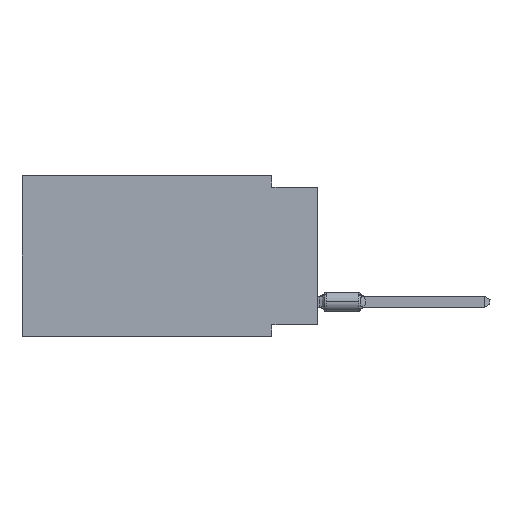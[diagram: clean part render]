
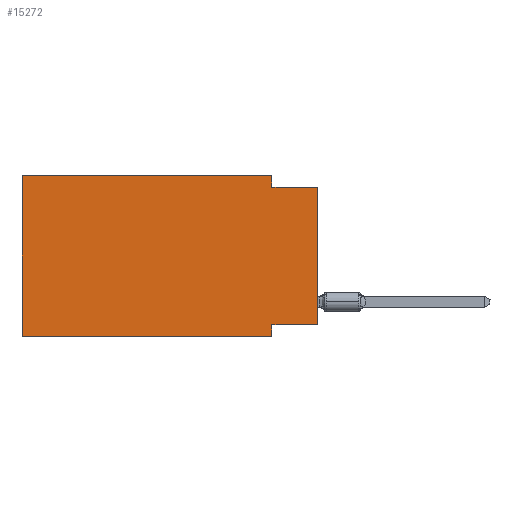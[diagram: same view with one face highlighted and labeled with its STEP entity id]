
A CAD part, left-side view. The second image highlights one B-rep face of the part: STEP entity #15272.
In plain terms, the highlighted planar face has unit normal (-1, 0, 0).
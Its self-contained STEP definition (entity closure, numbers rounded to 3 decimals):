
#421 = VECTOR ( 'NONE', #10780, 1000. ) ;
#685 = EDGE_CURVE ( 'NONE', #40255, #81278, #8906, .T. ) ;
#837 = ORIENTED_EDGE ( 'NONE', *, *, #5500, .F. ) ;
#1080 = VECTOR ( 'NONE', #57625, 1000. ) ;
#1341 = CARTESIAN_POINT ( 'NONE',  ( 0., 16.383, 0. ) ) ;
#1857 = ORIENTED_EDGE ( 'NONE', *, *, #63757, .F. ) ;
#5443 = DIRECTION ( 'NONE',  ( 0., 0., -1. ) ) ;
#5500 = EDGE_CURVE ( 'NONE', #42825, #16115, #10293, .T. ) ;
#5603 = ORIENTED_EDGE ( 'NONE', *, *, #50861, .F. ) ;
#8316 = CARTESIAN_POINT ( 'NONE',  ( 0., 2.54, 0. ) ) ;
#8602 = VERTEX_POINT ( 'NONE', #22568 ) ;
#8906 = LINE ( 'NONE', #74865, #79768 ) ;
#9498 = CARTESIAN_POINT ( 'NONE',  ( 0., 0., -0.635 ) ) ;
#9605 = LINE ( 'NONE', #62255, #16427 ) ;
#10293 = LINE ( 'NONE', #34338, #1080 ) ;
#10780 = DIRECTION ( 'NONE',  ( 0., -1., 0. ) ) ;
#15272 = ADVANCED_FACE ( 'NONE', ( #87398 ), #25463, .F. ) ;
#16115 = VERTEX_POINT ( 'NONE', #8316 ) ;
#16427 = VECTOR ( 'NONE', #29941, 1000. ) ;
#18495 = EDGE_LOOP ( 'NONE', ( #78484, #5603, #85163, #837, #1857, #58235, #41734, #46687 ) ) ;
#18888 = EDGE_CURVE ( 'NONE', #16115, #8602, #66050, .T. ) ;
#22229 = VECTOR ( 'NONE', #38894, 1000. ) ;
#22568 = CARTESIAN_POINT ( 'NONE',  ( 0., 2.54, -0.635 ) ) ;
#24429 = LINE ( 'NONE', #30181, #49712 ) ;
#25388 = CARTESIAN_POINT ( 'NONE',  ( 0., 16.383, -8.89 ) ) ;
#25463 = PLANE ( 'NONE',  #67395 ) ;
#25791 = CARTESIAN_POINT ( 'NONE',  ( 0., 2.54, 0. ) ) ;
#26759 = CARTESIAN_POINT ( 'NONE',  ( 0., 16.383, 0. ) ) ;
#28248 = VERTEX_POINT ( 'NONE', #60324 ) ;
#29941 = DIRECTION ( 'NONE',  ( 0., -1., 0. ) ) ;
#30181 = CARTESIAN_POINT ( 'NONE',  ( 0., 2.54, -8.89 ) ) ;
#31250 = EDGE_CURVE ( 'NONE', #40255, #40863, #35961, .T. ) ;
#32344 = CARTESIAN_POINT ( 'NONE',  ( 0., 2.54, -8.255 ) ) ;
#34338 = CARTESIAN_POINT ( 'NONE',  ( 0., 16.383, 0. ) ) ;
#35649 = EDGE_CURVE ( 'NONE', #77591, #28248, #86028, .T. ) ;
#35961 = LINE ( 'NONE', #76248, #59464 ) ;
#38894 = DIRECTION ( 'NONE',  ( 0., 0., 1. ) ) ;
#39158 = DIRECTION ( 'NONE',  ( 1., 0., 0. ) ) ;
#40255 = VERTEX_POINT ( 'NONE', #41470 ) ;
#40863 = VERTEX_POINT ( 'NONE', #9498 ) ;
#41470 = CARTESIAN_POINT ( 'NONE',  ( 0., 0., -8.255 ) ) ;
#41734 = ORIENTED_EDGE ( 'NONE', *, *, #46578, .F. ) ;
#42825 = VERTEX_POINT ( 'NONE', #1341 ) ;
#46578 = EDGE_CURVE ( 'NONE', #81278, #28248, #24429, .T. ) ;
#46687 = ORIENTED_EDGE ( 'NONE', *, *, #685, .F. ) ;
#49712 = VECTOR ( 'NONE', #57174, 1000. ) ;
#50861 = EDGE_CURVE ( 'NONE', #8602, #40863, #9605, .T. ) ;
#52436 = DIRECTION ( 'NONE',  ( 0., 0., -1. ) ) ;
#54940 = DIRECTION ( 'NONE',  ( 0., 1., 0. ) ) ;
#57174 = DIRECTION ( 'NONE',  ( 0., 0., -1. ) ) ;
#57185 = DIRECTION ( 'NONE',  ( 0., 0., 1. ) ) ;
#57625 = DIRECTION ( 'NONE',  ( 0., -1., 0. ) ) ;
#58235 = ORIENTED_EDGE ( 'NONE', *, *, #35649, .T. ) ;
#59464 = VECTOR ( 'NONE', #57185, 1000. ) ;
#60324 = CARTESIAN_POINT ( 'NONE',  ( 0., 2.54, -8.89 ) ) ;
#62255 = CARTESIAN_POINT ( 'NONE',  ( 0., 0., -0.635 ) ) ;
#63757 = EDGE_CURVE ( 'NONE', #77591, #42825, #65458, .T. ) ;
#65458 = LINE ( 'NONE', #79206, #22229 ) ;
#66050 = LINE ( 'NONE', #25791, #75154 ) ;
#67395 = AXIS2_PLACEMENT_3D ( 'NONE', #26759, #39158, #52436 ) ;
#74865 = CARTESIAN_POINT ( 'NONE',  ( 0., 0., -8.255 ) ) ;
#75154 = VECTOR ( 'NONE', #5443, 1000. ) ;
#76248 = CARTESIAN_POINT ( 'NONE',  ( 0., 0., 0. ) ) ;
#76794 = CARTESIAN_POINT ( 'NONE',  ( 0., 16.383, -8.89 ) ) ;
#77591 = VERTEX_POINT ( 'NONE', #76794 ) ;
#78484 = ORIENTED_EDGE ( 'NONE', *, *, #31250, .T. ) ;
#79206 = CARTESIAN_POINT ( 'NONE',  ( 0., 16.383, 0. ) ) ;
#79768 = VECTOR ( 'NONE', #54940, 1000. ) ;
#81278 = VERTEX_POINT ( 'NONE', #32344 ) ;
#85163 = ORIENTED_EDGE ( 'NONE', *, *, #18888, .F. ) ;
#86028 = LINE ( 'NONE', #25388, #421 ) ;
#87398 = FACE_OUTER_BOUND ( 'NONE', #18495, .T. ) ;
